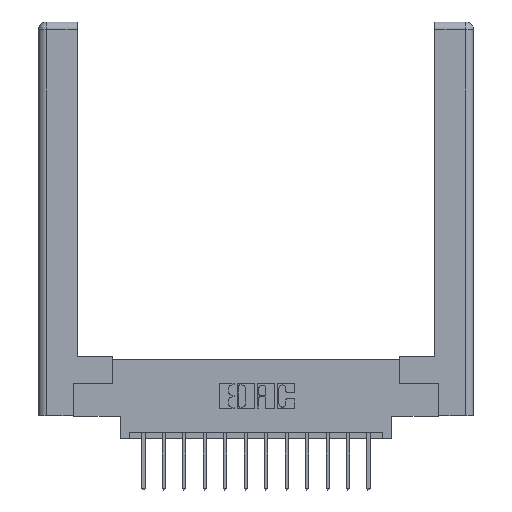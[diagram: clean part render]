
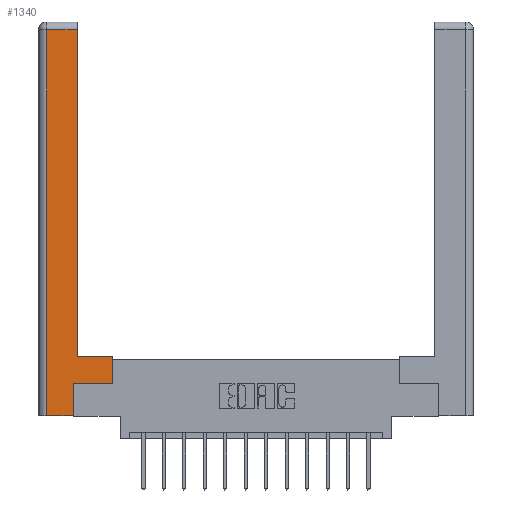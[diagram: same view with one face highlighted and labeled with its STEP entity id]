
A CAD part, top view. The second image highlights one B-rep face of the part: STEP entity #1340.
In plain terms, the highlighted planar face has unit normal (0, 0, 1).
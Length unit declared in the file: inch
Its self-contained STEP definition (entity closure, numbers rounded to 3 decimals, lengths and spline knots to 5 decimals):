
#40 = CARTESIAN_POINT ( 'NONE',  ( 0.0615, 0., 0. ) ) ;
#62 = AXIS2_PLACEMENT_3D ( 'NONE', #13872, #982, #8282 ) ;
#64 = EDGE_CURVE ( 'NONE', #8904, #5819, #4352, .T. ) ;
#280 = ORIENTED_EDGE ( 'NONE', *, *, #5525, .T. ) ;
#432 = EDGE_CURVE ( 'NONE', #5819, #10683, #639, .T. ) ;
#580 = CARTESIAN_POINT ( 'NONE',  ( 0.565, 0.45, 0. ) ) ;
#601 = CARTESIAN_POINT ( 'NONE',  ( 0.0615, 2.94, 0. ) ) ;
#639 = LINE ( 'NONE', #1134, #11259 ) ;
#982 = DIRECTION ( 'NONE',  ( 0., 0., -1. ) ) ;
#1037 = EDGE_CURVE ( 'NONE', #10683, #10652, #13370, .T. ) ;
#1134 = CARTESIAN_POINT ( 'NONE',  ( 0.295, 3., 0. ) ) ;
#1340 = ADVANCED_FACE ( 'NONE', ( #7002 ), #11380, .F. ) ;
#1579 = VECTOR ( 'NONE', #14367, 39.37008 ) ;
#1706 = DIRECTION ( 'NONE',  ( -1., 0., 0. ) ) ;
#1808 = DIRECTION ( 'NONE',  ( 1., 0., 0. ) ) ;
#1865 = VERTEX_POINT ( 'NONE', #9999 ) ;
#2122 = DIRECTION ( 'NONE',  ( 0., 1., 0. ) ) ;
#2246 = EDGE_CURVE ( 'NONE', #8701, #8904, #3135, .T. ) ;
#2310 = ORIENTED_EDGE ( 'NONE', *, *, #7658, .T. ) ;
#3135 = LINE ( 'NONE', #12036, #14480 ) ;
#3161 = DIRECTION ( 'NONE',  ( 0., 1., 0. ) ) ;
#3216 = VECTOR ( 'NONE', #3161, 39.37008 ) ;
#3700 = DIRECTION ( 'NONE',  ( 0., 1., 0. ) ) ;
#4352 = LINE ( 'NONE', #7192, #14358 ) ;
#4528 = LINE ( 'NONE', #5595, #14350 ) ;
#5080 = ORIENTED_EDGE ( 'NONE', *, *, #14978, .T. ) ;
#5473 = EDGE_LOOP ( 'NONE', ( #11029, #6863, #280, #5080, #12995, #2310, #14510, #6435 ) ) ;
#5525 = EDGE_CURVE ( 'NONE', #10652, #10362, #10198, .T. ) ;
#5595 = CARTESIAN_POINT ( 'NONE',  ( 0.565, 0.245, 0. ) ) ;
#5819 = VERTEX_POINT ( 'NONE', #9919 ) ;
#6435 = ORIENTED_EDGE ( 'NONE', *, *, #64, .T. ) ;
#6863 = ORIENTED_EDGE ( 'NONE', *, *, #1037, .T. ) ;
#7002 = FACE_OUTER_BOUND ( 'NONE', #5473, .T. ) ;
#7192 = CARTESIAN_POINT ( 'NONE',  ( 0.295, 0.45, 0. ) ) ;
#7345 = DIRECTION ( 'NONE',  ( -1., 0., 0. ) ) ;
#7440 = CARTESIAN_POINT ( 'NONE',  ( 0.0615, 0., 0. ) ) ;
#7658 = EDGE_CURVE ( 'NONE', #9571, #8701, #4528, .T. ) ;
#8143 = LINE ( 'NONE', #12712, #1579 ) ;
#8176 = VECTOR ( 'NONE', #1706, 39.37008 ) ;
#8257 = VECTOR ( 'NONE', #12460, 39.37008 ) ;
#8282 = DIRECTION ( 'NONE',  ( -1., 0., 0. ) ) ;
#8701 = VERTEX_POINT ( 'NONE', #14615 ) ;
#8904 = VERTEX_POINT ( 'NONE', #580 ) ;
#9043 = CARTESIAN_POINT ( 'NONE',  ( 0.0615, 2.94, 0. ) ) ;
#9571 = VERTEX_POINT ( 'NONE', #15075 ) ;
#9919 = CARTESIAN_POINT ( 'NONE',  ( 0.295, 0.45, 0. ) ) ;
#9999 = CARTESIAN_POINT ( 'NONE',  ( 0.265, 0., 0. ) ) ;
#10198 = LINE ( 'NONE', #7440, #8257 ) ;
#10362 = VERTEX_POINT ( 'NONE', #40 ) ;
#10512 = CARTESIAN_POINT ( 'NONE',  ( 0.265, 0.245, 0. ) ) ;
#10652 = VERTEX_POINT ( 'NONE', #9043 ) ;
#10683 = VERTEX_POINT ( 'NONE', #12779 ) ;
#10907 = LINE ( 'NONE', #10512, #3216 ) ;
#11029 = ORIENTED_EDGE ( 'NONE', *, *, #432, .T. ) ;
#11259 = VECTOR ( 'NONE', #3700, 39.37008 ) ;
#11380 = PLANE ( 'NONE',  #62 ) ;
#11899 = EDGE_CURVE ( 'NONE', #1865, #9571, #10907, .T. ) ;
#12036 = CARTESIAN_POINT ( 'NONE',  ( 0.565, 0.45, 0. ) ) ;
#12460 = DIRECTION ( 'NONE',  ( 0., -1., 0. ) ) ;
#12712 = CARTESIAN_POINT ( 'NONE',  ( 0.265, 0., 0. ) ) ;
#12779 = CARTESIAN_POINT ( 'NONE',  ( 0.295, 2.94, 0. ) ) ;
#12995 = ORIENTED_EDGE ( 'NONE', *, *, #11899, .T. ) ;
#13370 = LINE ( 'NONE', #601, #8176 ) ;
#13872 = CARTESIAN_POINT ( 'NONE',  ( 0., 0., 0. ) ) ;
#14350 = VECTOR ( 'NONE', #1808, 39.37008 ) ;
#14358 = VECTOR ( 'NONE', #7345, 39.37008 ) ;
#14367 = DIRECTION ( 'NONE',  ( 1., 0., 0. ) ) ;
#14480 = VECTOR ( 'NONE', #2122, 39.37008 ) ;
#14510 = ORIENTED_EDGE ( 'NONE', *, *, #2246, .T. ) ;
#14615 = CARTESIAN_POINT ( 'NONE',  ( 0.565, 0.245, 0. ) ) ;
#14978 = EDGE_CURVE ( 'NONE', #10362, #1865, #8143, .T. ) ;
#15075 = CARTESIAN_POINT ( 'NONE',  ( 0.265, 0.245, 0. ) ) ;
